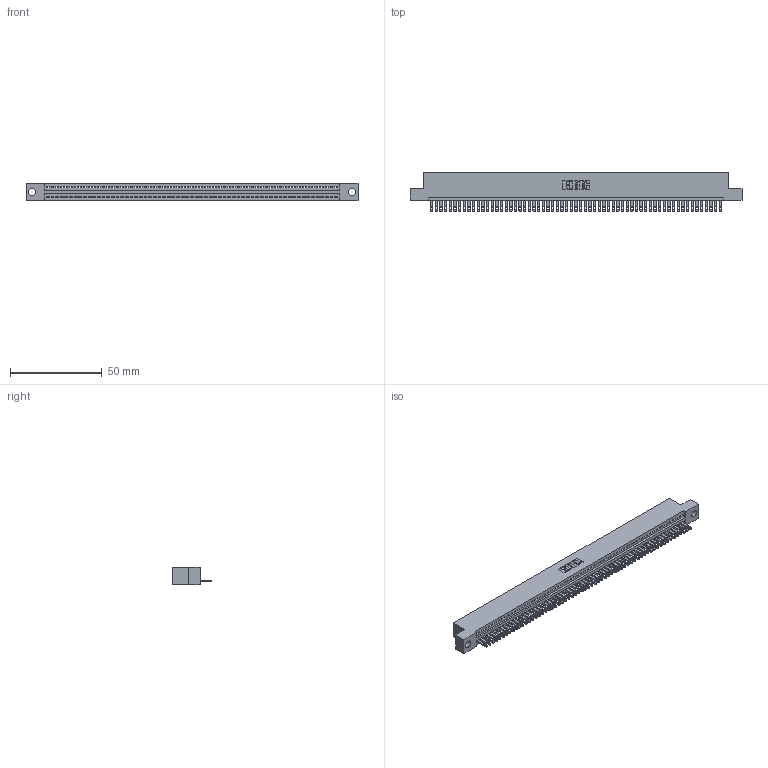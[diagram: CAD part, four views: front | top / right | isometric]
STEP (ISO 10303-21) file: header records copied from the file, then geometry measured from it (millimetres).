
FILE_DESCRIPTION (( 'STEP AP203' ), '1' );
FILE_NAME ('895-063-500-104.STEP', '2020-09-28T08:29:20', ( '' ), ( '' ), 'SwSTEP 2.0', 'SolidWorks 2020', '' );
FILE_SCHEMA (( 'CONFIG_CONTROL_DESIGN' ));
Length unit declared in the file: inch
Products named in the file (3): 895-063-500-104; 345-292-001_345-293-100; 845 Part_Flush Mounting Lugs - 0.156 Dia-TH
Assembly tree (64 placements, depth 2):
  895-063-500-104
    845 Part_Flush Mounting Lugs - 0.156 Dia-TH
    345-292-001_345-293-100  x63
Bounding box: 181.23 x 21.51 x 9.4 mm (x, y, z)
Volume: 17336.5 mm3; surface area: 23274.3 mm2
Topology: 64 solids, 64 shells, 3528 faces, 10925 edges, 7282 vertices
Faces by surface type: plane 2222, cylinder 1306
Entity records: 44521 total; most frequent: CARTESIAN_POINT 7717, ORIENTED_EDGE 7714, DIRECTION 6711, EDGE_CURVE 3857, VECTOR 3469, LINE 3469, VERTEX_POINT 2570, AXIS2_PLACEMENT_3D 1621
